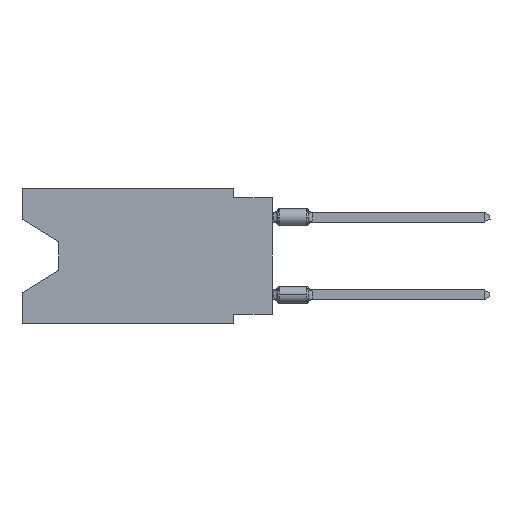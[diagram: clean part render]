
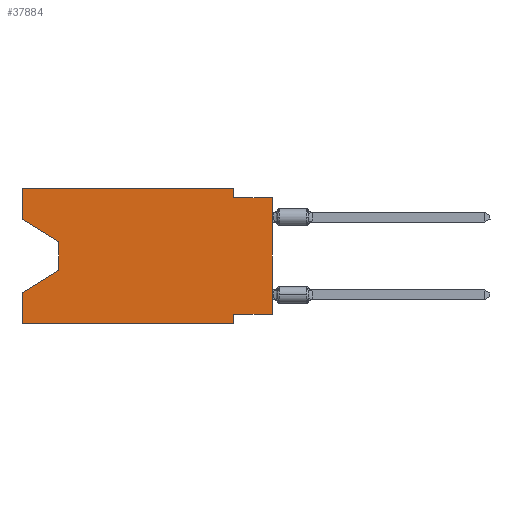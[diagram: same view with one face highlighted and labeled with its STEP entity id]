
A CAD part, left-side view. The second image highlights one B-rep face of the part: STEP entity #37884.
In plain terms, the highlighted planar face has unit normal (-1, 0, 0).
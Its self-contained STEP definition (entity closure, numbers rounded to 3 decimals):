
#390 = VERTEX_POINT ( 'NONE', #23872 ) ;
#1594 = ORIENTED_EDGE ( 'NONE', *, *, #20525, .F. ) ;
#1850 = CARTESIAN_POINT ( 'NONE',  ( 0., 16.383, -8.89 ) ) ;
#1878 = CARTESIAN_POINT ( 'NONE',  ( 0., 0., -0.635 ) ) ;
#2076 = LINE ( 'NONE', #1878, #16598 ) ;
#2305 = DIRECTION ( 'NONE',  ( 0., 0., 1. ) ) ;
#2458 = LINE ( 'NONE', #39697, #10715 ) ;
#2930 = CARTESIAN_POINT ( 'NONE',  ( 0., 2.54, -0.635 ) ) ;
#3388 = CARTESIAN_POINT ( 'NONE',  ( 0., 0., -0.635 ) ) ;
#3798 = VERTEX_POINT ( 'NONE', #2930 ) ;
#4490 = EDGE_CURVE ( 'NONE', #39632, #35411, #2458, .T. ) ;
#4538 = VECTOR ( 'NONE', #14185, 1000. ) ;
#4738 = LINE ( 'NONE', #26089, #30708 ) ;
#5001 = EDGE_CURVE ( 'NONE', #15174, #3798, #4738, .T. ) ;
#5137 = AXIS2_PLACEMENT_3D ( 'NONE', #17361, #26993, #17553 ) ;
#5305 = CARTESIAN_POINT ( 'NONE',  ( 0., 0., 0. ) ) ;
#5784 = VERTEX_POINT ( 'NONE', #3388 ) ;
#5950 = DIRECTION ( 'NONE',  ( 0., 0., 1. ) ) ;
#6115 = VECTOR ( 'NONE', #14313, 1000. ) ;
#7447 = ORIENTED_EDGE ( 'NONE', *, *, #38827, .T. ) ;
#7716 = DIRECTION ( 'NONE',  ( 0., -1., 0. ) ) ;
#8088 = DIRECTION ( 'NONE',  ( 0., -1., 0. ) ) ;
#8266 = CARTESIAN_POINT ( 'NONE',  ( 0., 16.383, -8.89 ) ) ;
#8730 = EDGE_CURVE ( 'NONE', #17891, #12801, #20470, .T. ) ;
#9381 = EDGE_CURVE ( 'NONE', #17891, #5784, #36316, .T. ) ;
#9602 = CARTESIAN_POINT ( 'NONE',  ( 0., 13.97, -3.505 ) ) ;
#10715 = VECTOR ( 'NONE', #32669, 1000. ) ;
#11346 = CARTESIAN_POINT ( 'NONE',  ( 0., 13.97, -5.385 ) ) ;
#12094 = EDGE_CURVE ( 'NONE', #16306, #18124, #36980, .T. ) ;
#12801 = VERTEX_POINT ( 'NONE', #16788 ) ;
#13384 = VECTOR ( 'NONE', #29026, 1000. ) ;
#13689 = VECTOR ( 'NONE', #5950, 1000. ) ;
#13984 = CARTESIAN_POINT ( 'NONE',  ( 0., 16.383, -2.038 ) ) ;
#14167 = CARTESIAN_POINT ( 'NONE',  ( 0., 16.383, 0. ) ) ;
#14185 = DIRECTION ( 'NONE',  ( 0., -0.855, -0.519 ) ) ;
#14313 = DIRECTION ( 'NONE',  ( 0., 0., 1. ) ) ;
#14712 = PLANE ( 'NONE',  #5137 ) ;
#15174 = VERTEX_POINT ( 'NONE', #28826 ) ;
#15625 = LINE ( 'NONE', #39796, #28467 ) ;
#15859 = EDGE_CURVE ( 'NONE', #22030, #15174, #29481, .T. ) ;
#16306 = VERTEX_POINT ( 'NONE', #8266 ) ;
#16371 = EDGE_CURVE ( 'NONE', #16306, #30284, #23592, .T. ) ;
#16598 = VECTOR ( 'NONE', #8088, 1000. ) ;
#16788 = CARTESIAN_POINT ( 'NONE',  ( 0., 2.54, -8.255 ) ) ;
#17361 = CARTESIAN_POINT ( 'NONE',  ( 0., 16.383, 0. ) ) ;
#17444 = CARTESIAN_POINT ( 'NONE',  ( 0., 0., -8.255 ) ) ;
#17551 = CARTESIAN_POINT ( 'NONE',  ( 0., 16.383, 0. ) ) ;
#17553 = DIRECTION ( 'NONE',  ( 0., 0., -1. ) ) ;
#17891 = VERTEX_POINT ( 'NONE', #23479 ) ;
#18124 = VERTEX_POINT ( 'NONE', #22987 ) ;
#19518 = ORIENTED_EDGE ( 'NONE', *, *, #4490, .T. ) ;
#20470 = LINE ( 'NONE', #17444, #29579 ) ;
#20525 = EDGE_CURVE ( 'NONE', #12801, #30284, #15625, .T. ) ;
#21190 = ORIENTED_EDGE ( 'NONE', *, *, #8730, .F. ) ;
#21875 = CARTESIAN_POINT ( 'NONE',  ( 0., 16.383, 0. ) ) ;
#22030 = VERTEX_POINT ( 'NONE', #29526 ) ;
#22354 = EDGE_LOOP ( 'NONE', ( #38817, #19518, #7447, #28808, #35128, #1594, #21190, #23009, #32608, #33224, #39561, #36008 ) ) ;
#22486 = DIRECTION ( 'NONE',  ( 0., 0., -1. ) ) ;
#22856 = EDGE_CURVE ( 'NONE', #390, #22030, #38896, .T. ) ;
#22987 = CARTESIAN_POINT ( 'NONE',  ( 0., 16.383, -6.852 ) ) ;
#23009 = ORIENTED_EDGE ( 'NONE', *, *, #9381, .T. ) ;
#23479 = CARTESIAN_POINT ( 'NONE',  ( 0., 0., -8.255 ) ) ;
#23592 = LINE ( 'NONE', #1850, #13384 ) ;
#23825 = VECTOR ( 'NONE', #2305, 1000. ) ;
#23872 = CARTESIAN_POINT ( 'NONE',  ( 0., 16.383, -2.038 ) ) ;
#24290 = DIRECTION ( 'NONE',  ( 0., 0., -1. ) ) ;
#26065 = LINE ( 'NONE', #13984, #4538 ) ;
#26089 = CARTESIAN_POINT ( 'NONE',  ( 0., 2.54, 0. ) ) ;
#26993 = DIRECTION ( 'NONE',  ( 1., 0., 0. ) ) ;
#27390 = FACE_OUTER_BOUND ( 'NONE', #22354, .T. ) ;
#28467 = VECTOR ( 'NONE', #24290, 1000. ) ;
#28808 = ORIENTED_EDGE ( 'NONE', *, *, #12094, .F. ) ;
#28815 = EDGE_CURVE ( 'NONE', #3798, #5784, #2076, .T. ) ;
#28826 = CARTESIAN_POINT ( 'NONE',  ( 0., 2.54, 0. ) ) ;
#29026 = DIRECTION ( 'NONE',  ( 0., -1., 0. ) ) ;
#29481 = LINE ( 'NONE', #14167, #33930 ) ;
#29526 = CARTESIAN_POINT ( 'NONE',  ( 0., 16.383, 0. ) ) ;
#29579 = VECTOR ( 'NONE', #29707, 1000. ) ;
#29707 = DIRECTION ( 'NONE',  ( 0., 1., 0. ) ) ;
#30284 = VERTEX_POINT ( 'NONE', #37355 ) ;
#30512 = CARTESIAN_POINT ( 'NONE',  ( 0., 13.97, -5.385 ) ) ;
#30708 = VECTOR ( 'NONE', #22486, 1000. ) ;
#31108 = LINE ( 'NONE', #30512, #34146 ) ;
#32608 = ORIENTED_EDGE ( 'NONE', *, *, #28815, .F. ) ;
#32669 = DIRECTION ( 'NONE',  ( 0., 0., -1. ) ) ;
#33224 = ORIENTED_EDGE ( 'NONE', *, *, #5001, .F. ) ;
#33930 = VECTOR ( 'NONE', #7716, 1000. ) ;
#34146 = VECTOR ( 'NONE', #36761, 1000. ) ;
#35128 = ORIENTED_EDGE ( 'NONE', *, *, #16371, .T. ) ;
#35411 = VERTEX_POINT ( 'NONE', #11346 ) ;
#36008 = ORIENTED_EDGE ( 'NONE', *, *, #22856, .F. ) ;
#36316 = LINE ( 'NONE', #5305, #23825 ) ;
#36761 = DIRECTION ( 'NONE',  ( 0., 0.855, -0.519 ) ) ;
#36908 = EDGE_CURVE ( 'NONE', #390, #39632, #26065, .T. ) ;
#36980 = LINE ( 'NONE', #21875, #13689 ) ;
#37355 = CARTESIAN_POINT ( 'NONE',  ( 0., 2.54, -8.89 ) ) ;
#37884 = ADVANCED_FACE ( 'NONE', ( #27390 ), #14712, .F. ) ;
#38817 = ORIENTED_EDGE ( 'NONE', *, *, #36908, .T. ) ;
#38827 = EDGE_CURVE ( 'NONE', #35411, #18124, #31108, .T. ) ;
#38896 = LINE ( 'NONE', #17551, #6115 ) ;
#39561 = ORIENTED_EDGE ( 'NONE', *, *, #15859, .F. ) ;
#39632 = VERTEX_POINT ( 'NONE', #9602 ) ;
#39697 = CARTESIAN_POINT ( 'NONE',  ( 0., 13.97, -3.505 ) ) ;
#39796 = CARTESIAN_POINT ( 'NONE',  ( 0., 2.54, -8.89 ) ) ;
